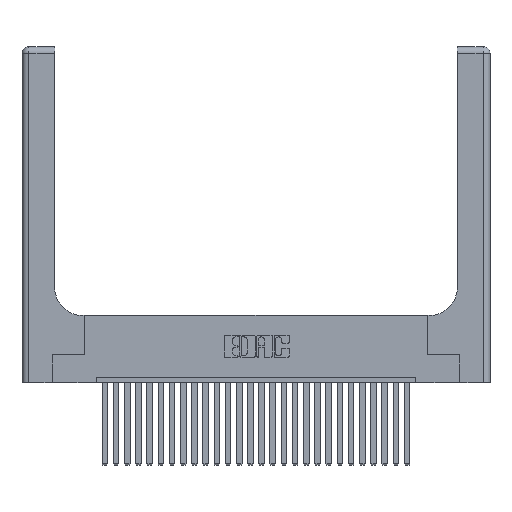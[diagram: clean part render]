
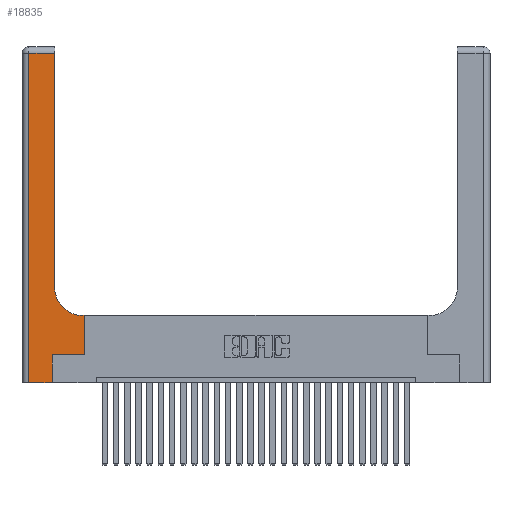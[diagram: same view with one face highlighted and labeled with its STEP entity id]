
A CAD part, top view. The second image highlights one B-rep face of the part: STEP entity #18835.
In plain terms, the highlighted planar face has unit normal (0, 0, 1).
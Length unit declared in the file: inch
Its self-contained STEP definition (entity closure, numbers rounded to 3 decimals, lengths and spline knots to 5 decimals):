
#454 = VERTEX_POINT ( 'NONE', #24008 ) ;
#786 = ORIENTED_EDGE ( 'NONE', *, *, #4314, .T. ) ;
#980 = LINE ( 'NONE', #17792, #4396 ) ;
#1012 = CARTESIAN_POINT ( 'NONE',  ( 0.06, 2.94, 0.37 ) ) ;
#1046 = VECTOR ( 'NONE', #13526, 39.37008 ) ;
#1173 = DIRECTION ( 'NONE',  ( 0., 1., 0. ) ) ;
#1273 = DIRECTION ( 'NONE',  ( 0., 1., 0. ) ) ;
#2319 = ORIENTED_EDGE ( 'NONE', *, *, #9199, .T. ) ;
#2589 = DIRECTION ( 'NONE',  ( 1., 0., 0. ) ) ;
#2768 = LINE ( 'NONE', #19913, #1046 ) ;
#3091 = DIRECTION ( 'NONE',  ( 0., 1., 0. ) ) ;
#3548 = DIRECTION ( 'NONE',  ( -1., 0., 0. ) ) ;
#3706 = VERTEX_POINT ( 'NONE', #5773 ) ;
#3803 = AXIS2_PLACEMENT_3D ( 'NONE', #19521, #23866, #13478 ) ;
#4218 = CARTESIAN_POINT ( 'NONE',  ( 0.2915, 0.85, 0.37 ) ) ;
#4314 = EDGE_CURVE ( 'NONE', #15202, #11741, #9917, .T. ) ;
#4396 = VECTOR ( 'NONE', #2589, 39.37008 ) ;
#5016 = EDGE_CURVE ( 'NONE', #3706, #6391, #7493, .T. ) ;
#5626 = EDGE_CURVE ( 'NONE', #11741, #454, #10080, .T. ) ;
#5773 = CARTESIAN_POINT ( 'NONE',  ( 0.5585, 0.6, 0.37 ) ) ;
#5794 = CARTESIAN_POINT ( 'NONE',  ( 0., 0., 0.37 ) ) ;
#6155 = ORIENTED_EDGE ( 'NONE', *, *, #5016, .T. ) ;
#6391 = VERTEX_POINT ( 'NONE', #9985 ) ;
#7493 = LINE ( 'NONE', #27410, #15926 ) ;
#7584 = EDGE_LOOP ( 'NONE', ( #8146, #2319, #786, #20102, #16609, #9081, #17684, #6155, #11354 ) ) ;
#7785 = AXIS2_PLACEMENT_3D ( 'NONE', #17239, #11030, #10946 ) ;
#8146 = ORIENTED_EDGE ( 'NONE', *, *, #23889, .T. ) ;
#8338 = VERTEX_POINT ( 'NONE', #4218 ) ;
#8560 = VECTOR ( 'NONE', #21420, 39.37008 ) ;
#9081 = ORIENTED_EDGE ( 'NONE', *, *, #18934, .T. ) ;
#9199 = EDGE_CURVE ( 'NONE', #25898, #15202, #2768, .T. ) ;
#9387 = VECTOR ( 'NONE', #23049, 39.37008 ) ;
#9917 = LINE ( 'NONE', #21141, #8560 ) ;
#9985 = CARTESIAN_POINT ( 'NONE',  ( 0.5415, 0.6, 0.37 ) ) ;
#10080 = LINE ( 'NONE', #5794, #9387 ) ;
#10946 = DIRECTION ( 'NONE',  ( -1., 0., 0. ) ) ;
#11030 = DIRECTION ( 'NONE',  ( 0., 0., -1. ) ) ;
#11354 = ORIENTED_EDGE ( 'NONE', *, *, #20415, .T. ) ;
#11732 = CARTESIAN_POINT ( 'NONE',  ( 0.5585, 0.25, 0.37 ) ) ;
#11741 = VERTEX_POINT ( 'NONE', #27144 ) ;
#13478 = DIRECTION ( 'NONE',  ( 1., 0., 0. ) ) ;
#13526 = DIRECTION ( 'NONE',  ( -1., 0., 0. ) ) ;
#13603 = VECTOR ( 'NONE', #3091, 39.37008 ) ;
#14226 = CARTESIAN_POINT ( 'NONE',  ( 0.5585, 0.25, 0.37 ) ) ;
#14405 = CARTESIAN_POINT ( 'NONE',  ( 0.2915, 3., 0.37 ) ) ;
#15202 = VERTEX_POINT ( 'NONE', #1012 ) ;
#15926 = VECTOR ( 'NONE', #3548, 39.37008 ) ;
#16609 = ORIENTED_EDGE ( 'NONE', *, *, #22893, .T. ) ;
#17239 = CARTESIAN_POINT ( 'NONE',  ( 0., 3., 0.37 ) ) ;
#17684 = ORIENTED_EDGE ( 'NONE', *, *, #22412, .T. ) ;
#17792 = CARTESIAN_POINT ( 'NONE',  ( 0.269, 0.25, 0.37 ) ) ;
#17996 = VECTOR ( 'NONE', #1273, 39.37008 ) ;
#18305 = LINE ( 'NONE', #14405, #27414 ) ;
#18835 = ADVANCED_FACE ( 'NONE', ( #19888 ), #19402, .F. ) ;
#18934 = EDGE_CURVE ( 'NONE', #26410, #27365, #980, .T. ) ;
#19293 = CARTESIAN_POINT ( 'NONE',  ( 0.269, 0.25, 0.37 ) ) ;
#19402 = PLANE ( 'NONE',  #7785 ) ;
#19484 = CIRCLE ( 'NONE', #3803, 0.25 ) ;
#19521 = CARTESIAN_POINT ( 'NONE',  ( 0.5415, 0.85, 0.37 ) ) ;
#19888 = FACE_OUTER_BOUND ( 'NONE', #7584, .T. ) ;
#19913 = CARTESIAN_POINT ( 'NONE',  ( 0., 2.94, 0.37 ) ) ;
#20102 = ORIENTED_EDGE ( 'NONE', *, *, #5626, .T. ) ;
#20415 = EDGE_CURVE ( 'NONE', #6391, #8338, #19484, .T. ) ;
#21141 = CARTESIAN_POINT ( 'NONE',  ( 0.06, 3., 0.37 ) ) ;
#21420 = DIRECTION ( 'NONE',  ( 0., -1., 0. ) ) ;
#21808 = CARTESIAN_POINT ( 'NONE',  ( 0.269, 0., 0.37 ) ) ;
#22412 = EDGE_CURVE ( 'NONE', #27365, #3706, #23082, .T. ) ;
#22893 = EDGE_CURVE ( 'NONE', #454, #26410, #26100, .T. ) ;
#23049 = DIRECTION ( 'NONE',  ( 1., 0., 0. ) ) ;
#23082 = LINE ( 'NONE', #14226, #17996 ) ;
#23866 = DIRECTION ( 'NONE',  ( 0., 0., -1. ) ) ;
#23889 = EDGE_CURVE ( 'NONE', #8338, #25898, #18305, .T. ) ;
#24008 = CARTESIAN_POINT ( 'NONE',  ( 0.269, 0., 0.37 ) ) ;
#25898 = VERTEX_POINT ( 'NONE', #27060 ) ;
#26100 = LINE ( 'NONE', #21808, #13603 ) ;
#26410 = VERTEX_POINT ( 'NONE', #19293 ) ;
#27060 = CARTESIAN_POINT ( 'NONE',  ( 0.2915, 2.94, 0.37 ) ) ;
#27144 = CARTESIAN_POINT ( 'NONE',  ( 0.06, 0., 0.37 ) ) ;
#27365 = VERTEX_POINT ( 'NONE', #11732 ) ;
#27410 = CARTESIAN_POINT ( 'NONE',  ( 0.2915, 0.6, 0.37 ) ) ;
#27414 = VECTOR ( 'NONE', #1173, 39.37008 ) ;
